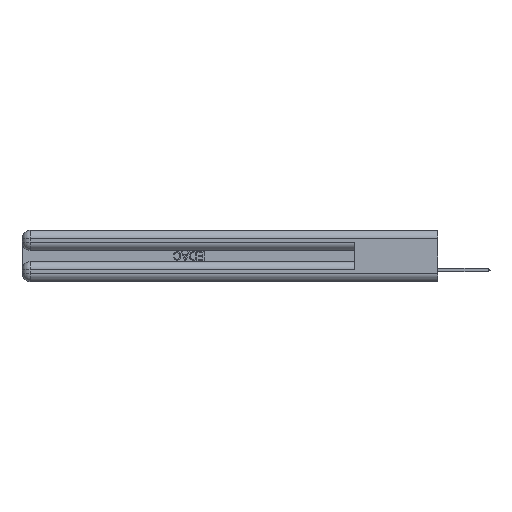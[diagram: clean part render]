
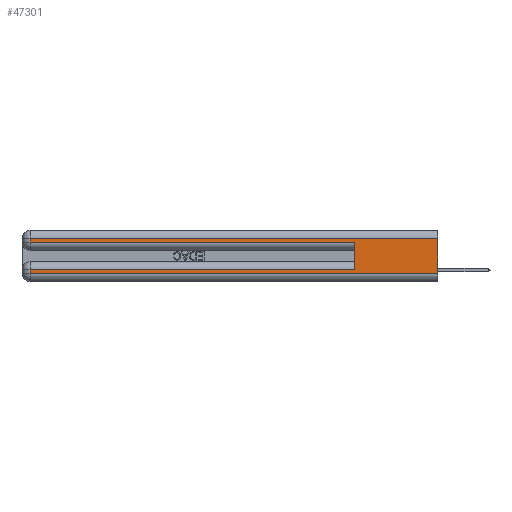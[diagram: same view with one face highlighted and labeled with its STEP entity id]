
A CAD part, left-side view. The second image highlights one B-rep face of the part: STEP entity #47301.
In plain terms, the highlighted planar face has unit normal (-1, 0, 0).
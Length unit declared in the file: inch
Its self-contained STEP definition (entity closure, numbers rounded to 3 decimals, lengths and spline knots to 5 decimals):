
#285 = VERTEX_POINT ( 'NONE', #36042 ) ;
#1216 = VECTOR ( 'NONE', #37023, 39.37008 ) ;
#2096 = CARTESIAN_POINT ( 'NONE',  ( 0., 0., 0.06 ) ) ;
#2231 = CARTESIAN_POINT ( 'NONE',  ( 0., 0.6, 0.145 ) ) ;
#2350 = VECTOR ( 'NONE', #10184, 39.37008 ) ;
#2420 = PLANE ( 'NONE',  #5903 ) ;
#3563 = LINE ( 'NONE', #10019, #2350 ) ;
#3710 = CARTESIAN_POINT ( 'NONE',  ( 0., 0.6, 0.085 ) ) ;
#4268 = LINE ( 'NONE', #32734, #28879 ) ;
#4300 = LINE ( 'NONE', #48685, #44002 ) ;
#5903 = AXIS2_PLACEMENT_3D ( 'NONE', #21251, #25443, #9987 ) ;
#6679 = LINE ( 'NONE', #2231, #1216 ) ;
#9420 = VERTEX_POINT ( 'NONE', #21238 ) ;
#9987 = DIRECTION ( 'NONE',  ( 0., 0., -1. ) ) ;
#10019 = CARTESIAN_POINT ( 'NONE',  ( 0., 0., 0.31 ) ) ;
#10184 = DIRECTION ( 'NONE',  ( 0., 1., 0. ) ) ;
#11761 = VECTOR ( 'NONE', #22543, 39.37008 ) ;
#13680 = LINE ( 'NONE', #43689, #20916 ) ;
#13876 = DIRECTION ( 'NONE',  ( 0., -1., 0. ) ) ;
#14200 = EDGE_CURVE ( 'NONE', #46355, #19128, #49688, .T. ) ;
#15055 = EDGE_CURVE ( 'NONE', #19128, #19280, #17102, .T. ) ;
#15298 = CARTESIAN_POINT ( 'NONE',  ( 0., 2.94, 0.37 ) ) ;
#15799 = CARTESIAN_POINT ( 'NONE',  ( 0., 0., 0.06 ) ) ;
#17102 = LINE ( 'NONE', #2096, #21341 ) ;
#17270 = DIRECTION ( 'NONE',  ( 0., 0., -1. ) ) ;
#17917 = DIRECTION ( 'NONE',  ( 0., -1., 0. ) ) ;
#17953 = VERTEX_POINT ( 'NONE', #3710 ) ;
#18585 = ORIENTED_EDGE ( 'NONE', *, *, #14200, .T. ) ;
#18990 = VERTEX_POINT ( 'NONE', #36549 ) ;
#19128 = VERTEX_POINT ( 'NONE', #20733 ) ;
#19280 = VERTEX_POINT ( 'NONE', #15799 ) ;
#20623 = DIRECTION ( 'NONE',  ( 0., 0., -1. ) ) ;
#20733 = CARTESIAN_POINT ( 'NONE',  ( 0., 2.94, 0.06 ) ) ;
#20916 = VECTOR ( 'NONE', #20623, 39.37008 ) ;
#21034 = VERTEX_POINT ( 'NONE', #21363 ) ;
#21105 = ORIENTED_EDGE ( 'NONE', *, *, #45827, .T. ) ;
#21238 = CARTESIAN_POINT ( 'NONE',  ( 0., 0.6, 0.285 ) ) ;
#21251 = CARTESIAN_POINT ( 'NONE',  ( 0., 0., 0.37 ) ) ;
#21341 = VECTOR ( 'NONE', #13876, 39.37008 ) ;
#21363 = CARTESIAN_POINT ( 'NONE',  ( 0., 2.94, 0.31 ) ) ;
#22543 = DIRECTION ( 'NONE',  ( 0., 0., -1. ) ) ;
#22748 = ORIENTED_EDGE ( 'NONE', *, *, #40149, .T. ) ;
#23676 = EDGE_CURVE ( 'NONE', #18990, #9420, #4300, .T. ) ;
#25443 = DIRECTION ( 'NONE',  ( 1., 0., 0. ) ) ;
#28271 = EDGE_CURVE ( 'NONE', #285, #21034, #3563, .T. ) ;
#28592 = EDGE_LOOP ( 'NONE', ( #39493, #36701, #22748, #29052, #37912, #21105, #18585, #37988 ) ) ;
#28879 = VECTOR ( 'NONE', #17270, 39.37008 ) ;
#29052 = ORIENTED_EDGE ( 'NONE', *, *, #23676, .T. ) ;
#31545 = LINE ( 'NONE', #40173, #39398 ) ;
#32734 = CARTESIAN_POINT ( 'NONE',  ( 0., 2.94, 0.37 ) ) ;
#36042 = CARTESIAN_POINT ( 'NONE',  ( 0., 0., 0.31 ) ) ;
#36128 = DIRECTION ( 'NONE',  ( 0., 1., 0. ) ) ;
#36549 = CARTESIAN_POINT ( 'NONE',  ( 0., 2.94, 0.285 ) ) ;
#36701 = ORIENTED_EDGE ( 'NONE', *, *, #28271, .T. ) ;
#37023 = DIRECTION ( 'NONE',  ( 0., 0., 1. ) ) ;
#37116 = CARTESIAN_POINT ( 'NONE',  ( 0., 2.94, 0.085 ) ) ;
#37912 = ORIENTED_EDGE ( 'NONE', *, *, #43002, .F. ) ;
#37988 = ORIENTED_EDGE ( 'NONE', *, *, #15055, .T. ) ;
#39029 = FACE_OUTER_BOUND ( 'NONE', #28592, .T. ) ;
#39398 = VECTOR ( 'NONE', #36128, 39.37008 ) ;
#39493 = ORIENTED_EDGE ( 'NONE', *, *, #44494, .F. ) ;
#40149 = EDGE_CURVE ( 'NONE', #21034, #18990, #4268, .T. ) ;
#40173 = CARTESIAN_POINT ( 'NONE',  ( 0., 0., 0.085 ) ) ;
#43002 = EDGE_CURVE ( 'NONE', #17953, #9420, #6679, .T. ) ;
#43689 = CARTESIAN_POINT ( 'NONE',  ( 0., 0., 0.37 ) ) ;
#44002 = VECTOR ( 'NONE', #17917, 39.37008 ) ;
#44494 = EDGE_CURVE ( 'NONE', #285, #19280, #13680, .T. ) ;
#45827 = EDGE_CURVE ( 'NONE', #17953, #46355, #31545, .T. ) ;
#46355 = VERTEX_POINT ( 'NONE', #37116 ) ;
#47301 = ADVANCED_FACE ( 'NONE', ( #39029 ), #2420, .F. ) ;
#48685 = CARTESIAN_POINT ( 'NONE',  ( 0., 0., 0.285 ) ) ;
#49688 = LINE ( 'NONE', #15298, #11761 ) ;
